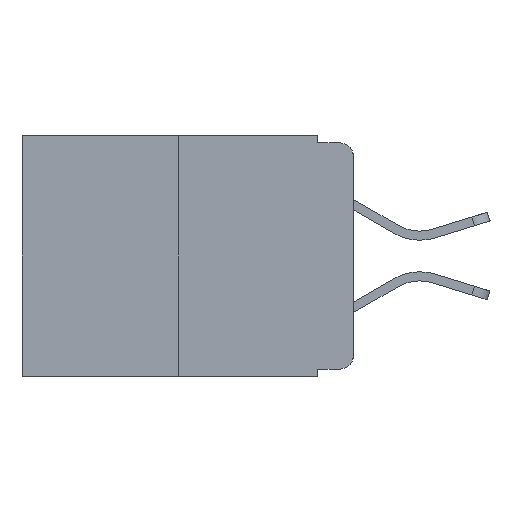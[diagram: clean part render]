
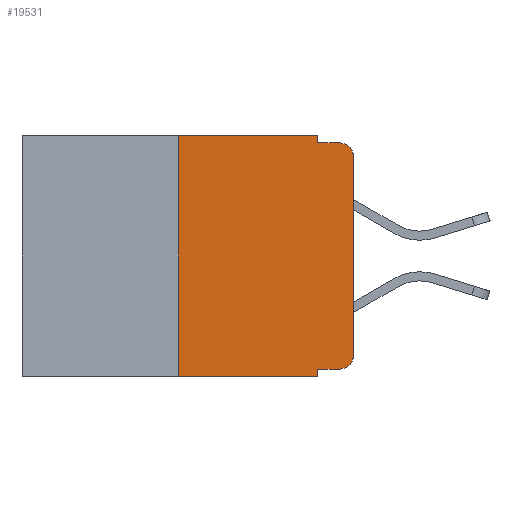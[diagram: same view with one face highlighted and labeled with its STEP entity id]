
A CAD part, left-side view. The second image highlights one B-rep face of the part: STEP entity #19531.
In plain terms, the highlighted planar face has unit normal (-1, 0, 0).
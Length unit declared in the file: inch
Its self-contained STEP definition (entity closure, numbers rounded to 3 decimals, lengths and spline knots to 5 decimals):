
#77 = EDGE_CURVE ( 'NONE', #15417, #15248, #3134, .T. ) ;
#87 = VERTEX_POINT ( 'NONE', #1413 ) ;
#129 = CARTESIAN_POINT ( 'NONE',  ( 0., 0.25, -0.343 ) ) ;
#327 = EDGE_LOOP ( 'NONE', ( #6071, #13345, #4073, #1766, #5369, #8390, #14127, #13423, #14410, #4675 ) ) ;
#333 = AXIS2_PLACEMENT_3D ( 'NONE', #20227, #6168, #17215 ) ;
#465 = VECTOR ( 'NONE', #5921, 39.37008 ) ;
#921 = VERTEX_POINT ( 'NONE', #16692 ) ;
#1198 = EDGE_CURVE ( 'NONE', #19719, #921, #3859, .T. ) ;
#1413 = CARTESIAN_POINT ( 'NONE',  ( 0., 0.02, -0.01 ) ) ;
#1761 = CARTESIAN_POINT ( 'NONE',  ( 0., 0., -0.313 ) ) ;
#1766 = ORIENTED_EDGE ( 'NONE', *, *, #2346, .F. ) ;
#1967 = CARTESIAN_POINT ( 'NONE',  ( 0., 0., -0.03 ) ) ;
#2115 = AXIS2_PLACEMENT_3D ( 'NONE', #5206, #16304, #6811 ) ;
#2173 = VECTOR ( 'NONE', #17160, 39.37008 ) ;
#2346 = EDGE_CURVE ( 'NONE', #14919, #20085, #13369, .T. ) ;
#2615 = VECTOR ( 'NONE', #3426, 39.37008 ) ;
#2910 = PLANE ( 'NONE',  #333 ) ;
#3134 = LINE ( 'NONE', #11149, #2615 ) ;
#3286 = CARTESIAN_POINT ( 'NONE',  ( 0., 0.051, -0.343 ) ) ;
#3426 = DIRECTION ( 'NONE',  ( 0., 0., -1. ) ) ;
#3591 = DIRECTION ( 'NONE',  ( 0., -1., 0. ) ) ;
#3771 = DIRECTION ( 'NONE',  ( 0., -1., 0. ) ) ;
#3859 = LINE ( 'NONE', #8829, #20115 ) ;
#3877 = DIRECTION ( 'NONE',  ( 0., 0., 1. ) ) ;
#4073 = ORIENTED_EDGE ( 'NONE', *, *, #4525, .F. ) ;
#4483 = LINE ( 'NONE', #11760, #4989 ) ;
#4525 = EDGE_CURVE ( 'NONE', #20085, #87, #4483, .T. ) ;
#4675 = ORIENTED_EDGE ( 'NONE', *, *, #17655, .T. ) ;
#4689 = CIRCLE ( 'NONE', #2115, 0.02 ) ;
#4989 = VECTOR ( 'NONE', #3771, 39.37008 ) ;
#5141 = CARTESIAN_POINT ( 'NONE',  ( 0., 0.473, 0. ) ) ;
#5206 = CARTESIAN_POINT ( 'NONE',  ( 0., 0.02, -0.03 ) ) ;
#5369 = ORIENTED_EDGE ( 'NONE', *, *, #14712, .F. ) ;
#5598 = EDGE_CURVE ( 'NONE', #20455, #87, #4689, .T. ) ;
#5683 = CARTESIAN_POINT ( 'NONE',  ( 0., 0.051, 0. ) ) ;
#5867 = CARTESIAN_POINT ( 'NONE',  ( 0., 0.051, -0.01 ) ) ;
#5921 = DIRECTION ( 'NONE',  ( 0., 0., -1. ) ) ;
#6071 = ORIENTED_EDGE ( 'NONE', *, *, #7730, .T. ) ;
#6168 = DIRECTION ( 'NONE',  ( 1., 0., 0. ) ) ;
#6500 = DIRECTION ( 'NONE',  ( -1., 0., 0. ) ) ;
#6811 = DIRECTION ( 'NONE',  ( 0., 0., -1. ) ) ;
#7364 = FACE_OUTER_BOUND ( 'NONE', #327, .T. ) ;
#7419 = CIRCLE ( 'NONE', #11852, 0.02 ) ;
#7730 = EDGE_CURVE ( 'NONE', #11773, #20455, #16794, .T. ) ;
#7886 = LINE ( 'NONE', #5141, #19910 ) ;
#8390 = ORIENTED_EDGE ( 'NONE', *, *, #1198, .F. ) ;
#8829 = CARTESIAN_POINT ( 'NONE',  ( 0., 0.25, 0. ) ) ;
#10880 = CARTESIAN_POINT ( 'NONE',  ( 0., 0.473, -0.343 ) ) ;
#11149 = CARTESIAN_POINT ( 'NONE',  ( 0., 0.051, 0. ) ) ;
#11760 = CARTESIAN_POINT ( 'NONE',  ( 0., 0.051, -0.01 ) ) ;
#11773 = VERTEX_POINT ( 'NONE', #1761 ) ;
#11852 = AXIS2_PLACEMENT_3D ( 'NONE', #15993, #6500, #17542 ) ;
#12150 = VECTOR ( 'NONE', #3877, 39.37008 ) ;
#12160 = DIRECTION ( 'NONE',  ( 0., 0., 1. ) ) ;
#12489 = DIRECTION ( 'NONE',  ( 0., -1., 0. ) ) ;
#13345 = ORIENTED_EDGE ( 'NONE', *, *, #5598, .T. ) ;
#13369 = LINE ( 'NONE', #18592, #465 ) ;
#13423 = ORIENTED_EDGE ( 'NONE', *, *, #77, .F. ) ;
#13466 = CARTESIAN_POINT ( 'NONE',  ( 0., 0., 0. ) ) ;
#14127 = ORIENTED_EDGE ( 'NONE', *, *, #16895, .T. ) ;
#14410 = ORIENTED_EDGE ( 'NONE', *, *, #18660, .T. ) ;
#14712 = EDGE_CURVE ( 'NONE', #921, #14919, #7886, .T. ) ;
#14919 = VERTEX_POINT ( 'NONE', #5683 ) ;
#15248 = VERTEX_POINT ( 'NONE', #3286 ) ;
#15417 = VERTEX_POINT ( 'NONE', #17892 ) ;
#15993 = CARTESIAN_POINT ( 'NONE',  ( 0., 0.02, -0.313 ) ) ;
#16062 = VECTOR ( 'NONE', #12489, 39.37008 ) ;
#16304 = DIRECTION ( 'NONE',  ( -1., 0., 0. ) ) ;
#16692 = CARTESIAN_POINT ( 'NONE',  ( 0., 0.25, 0. ) ) ;
#16794 = LINE ( 'NONE', #13466, #12150 ) ;
#16895 = EDGE_CURVE ( 'NONE', #19719, #15248, #18063, .T. ) ;
#17160 = DIRECTION ( 'NONE',  ( 0., -1., 0. ) ) ;
#17215 = DIRECTION ( 'NONE',  ( 0., 0., -1. ) ) ;
#17542 = DIRECTION ( 'NONE',  ( 0., 0., -1. ) ) ;
#17655 = EDGE_CURVE ( 'NONE', #19226, #11773, #7419, .T. ) ;
#17892 = CARTESIAN_POINT ( 'NONE',  ( 0., 0.051, -0.333 ) ) ;
#18063 = LINE ( 'NONE', #10880, #2173 ) ;
#18592 = CARTESIAN_POINT ( 'NONE',  ( 0., 0.051, 0. ) ) ;
#18660 = EDGE_CURVE ( 'NONE', #15417, #19226, #20126, .T. ) ;
#19226 = VERTEX_POINT ( 'NONE', #19454 ) ;
#19454 = CARTESIAN_POINT ( 'NONE',  ( 0., 0.02, -0.333 ) ) ;
#19531 = ADVANCED_FACE ( 'NONE', ( #7364 ), #2910, .F. ) ;
#19719 = VERTEX_POINT ( 'NONE', #129 ) ;
#19910 = VECTOR ( 'NONE', #3591, 39.37008 ) ;
#20085 = VERTEX_POINT ( 'NONE', #5867 ) ;
#20115 = VECTOR ( 'NONE', #12160, 39.37008 ) ;
#20126 = LINE ( 'NONE', #20171, #16062 ) ;
#20171 = CARTESIAN_POINT ( 'NONE',  ( 0., 0.051, -0.333 ) ) ;
#20227 = CARTESIAN_POINT ( 'NONE',  ( 0., 0.473, 0. ) ) ;
#20455 = VERTEX_POINT ( 'NONE', #1967 ) ;
